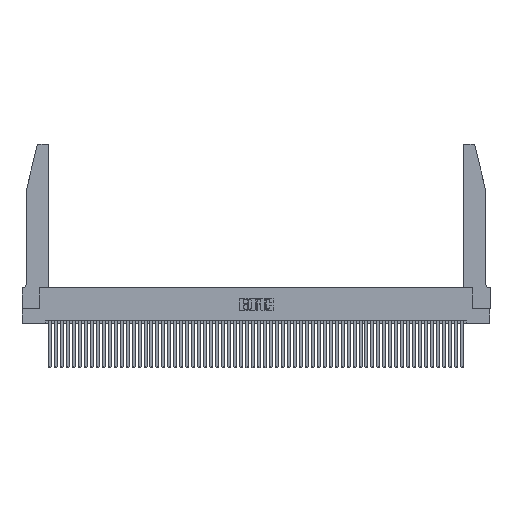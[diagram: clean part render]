
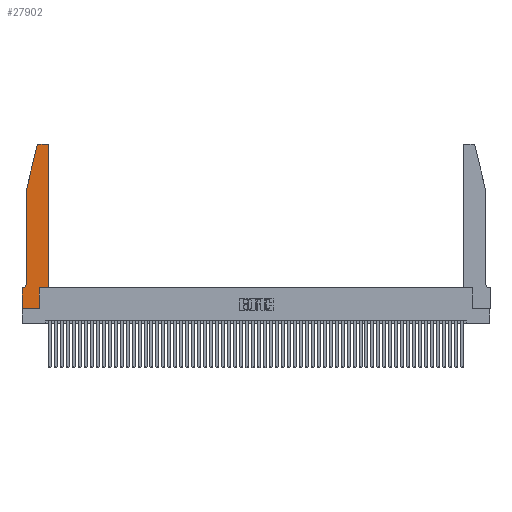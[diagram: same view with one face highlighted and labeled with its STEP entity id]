
A CAD part, top view. The second image highlights one B-rep face of the part: STEP entity #27902.
In plain terms, the highlighted planar face has unit normal (0, 0, 1).
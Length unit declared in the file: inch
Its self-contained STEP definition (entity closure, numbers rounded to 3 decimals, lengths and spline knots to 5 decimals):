
#57 = ORIENTED_EDGE ( 'NONE', *, *, #36650, .T. ) ;
#252 = DIRECTION ( 'NONE',  ( -1., 0., 0. ) ) ;
#535 = LINE ( 'NONE', #14785, #45060 ) ;
#554 = CARTESIAN_POINT ( 'NONE',  ( 0.284, 2.75, 0.37 ) ) ;
#903 = DIRECTION ( 'NONE',  ( 0., 0., 1. ) ) ;
#1165 = EDGE_CURVE ( 'NONE', #12063, #47447, #8140, .T. ) ;
#1200 = CARTESIAN_POINT ( 'NONE',  ( 0.0755, 2., 0.37 ) ) ;
#1361 = CARTESIAN_POINT ( 'NONE',  ( 0., 0.35, 0.37 ) ) ;
#1386 = FACE_OUTER_BOUND ( 'NONE', #52553, .T. ) ;
#3301 = DIRECTION ( 'NONE',  ( -1., 0., 0. ) ) ;
#3852 = CARTESIAN_POINT ( 'NONE',  ( 0.4505, 0.35, 0.37 ) ) ;
#4011 = VERTEX_POINT ( 'NONE', #37420 ) ;
#4111 = EDGE_CURVE ( 'NONE', #13767, #12063, #19401, .T. ) ;
#4223 = CARTESIAN_POINT ( 'NONE',  ( 0.0055, 0.35, 0.37 ) ) ;
#5656 = CARTESIAN_POINT ( 'NONE',  ( 0.2865, 0.35, 0.37 ) ) ;
#5822 = LINE ( 'NONE', #30712, #37590 ) ;
#6964 = VECTOR ( 'NONE', #34109, 39.37008 ) ;
#7444 = EDGE_CURVE ( 'NONE', #44826, #19031, #23081, .T. ) ;
#7683 = DIRECTION ( 'NONE',  ( 0., 0., 1. ) ) ;
#7916 = DIRECTION ( 'NONE',  ( 0., -1., 0. ) ) ;
#8140 = CIRCLE ( 'NONE', #15231, 0.03 ) ;
#8485 = DIRECTION ( 'NONE',  ( 0., 0., 1. ) ) ;
#9346 = ORIENTED_EDGE ( 'NONE', *, *, #47945, .T. ) ;
#9881 = LINE ( 'NONE', #29501, #21420 ) ;
#10178 = VECTOR ( 'NONE', #25687, 39.37008 ) ;
#10452 = VERTEX_POINT ( 'NONE', #23233 ) ;
#10533 = CIRCLE ( 'NONE', #49931, 0.03 ) ;
#10679 = CARTESIAN_POINT ( 'NONE',  ( 0.0755, 0.42, 0.37 ) ) ;
#11025 = LINE ( 'NONE', #46270, #55448 ) ;
#11802 = CARTESIAN_POINT ( 'NONE',  ( 0.4205, 2.75, 0.37 ) ) ;
#11993 = VERTEX_POINT ( 'NONE', #34749 ) ;
#12063 = VERTEX_POINT ( 'NONE', #554 ) ;
#13767 = VERTEX_POINT ( 'NONE', #11802 ) ;
#14785 = CARTESIAN_POINT ( 'NONE',  ( 0.4505, 0.35, 0.37 ) ) ;
#14830 = ORIENTED_EDGE ( 'NONE', *, *, #38845, .T. ) ;
#15144 = AXIS2_PLACEMENT_3D ( 'NONE', #34397, #8485, #38684 ) ;
#15231 = AXIS2_PLACEMENT_3D ( 'NONE', #33603, #7683, #37919 ) ;
#15746 = CARTESIAN_POINT ( 'NONE',  ( 0.4505, 2.72, 0.37 ) ) ;
#16103 = ORIENTED_EDGE ( 'NONE', *, *, #24331, .T. ) ;
#16432 = ORIENTED_EDGE ( 'NONE', *, *, #1165, .T. ) ;
#16572 = VECTOR ( 'NONE', #23095, 39.37008 ) ;
#19006 = ORIENTED_EDGE ( 'NONE', *, *, #34104, .T. ) ;
#19031 = VERTEX_POINT ( 'NONE', #29250 ) ;
#19401 = LINE ( 'NONE', #50860, #50999 ) ;
#20059 = EDGE_CURVE ( 'NONE', #19031, #11993, #28097, .T. ) ;
#21118 = EDGE_CURVE ( 'NONE', #48127, #44826, #11025, .T. ) ;
#21420 = VECTOR ( 'NONE', #7916, 39.37008 ) ;
#23081 = LINE ( 'NONE', #25513, #10178 ) ;
#23095 = DIRECTION ( 'NONE',  ( 0., 1., 0. ) ) ;
#23233 = CARTESIAN_POINT ( 'NONE',  ( 0.4505, 0.35, 0.37 ) ) ;
#23531 = DIRECTION ( 'NONE',  ( 1., 0., 0. ) ) ;
#23615 = VECTOR ( 'NONE', #48489, 39.37008 ) ;
#24331 = EDGE_CURVE ( 'NONE', #11993, #10452, #535, .T. ) ;
#25513 = CARTESIAN_POINT ( 'NONE',  ( 0., 0., 0.37 ) ) ;
#25687 = DIRECTION ( 'NONE',  ( 1., 0., 0. ) ) ;
#25731 = PLANE ( 'NONE',  #15144 ) ;
#26732 = VERTEX_POINT ( 'NONE', #10679 ) ;
#26828 = CARTESIAN_POINT ( 'NONE',  ( 0.4205, 2.72, 0.37 ) ) ;
#27902 = ADVANCED_FACE ( 'NONE', ( #1386 ), #25731, .T. ) ;
#28097 = LINE ( 'NONE', #5656, #16572 ) ;
#28155 = ORIENTED_EDGE ( 'NONE', *, *, #4111, .T. ) ;
#29241 = DIRECTION ( 'NONE',  ( 0., 0., -1. ) ) ;
#29250 = CARTESIAN_POINT ( 'NONE',  ( 0.2865, 0., 0.37 ) ) ;
#29501 = CARTESIAN_POINT ( 'NONE',  ( 0.0755, 2., 0.37 ) ) ;
#30712 = CARTESIAN_POINT ( 'NONE',  ( 0.0755, 0.35, 0.37 ) ) ;
#30975 = ORIENTED_EDGE ( 'NONE', *, *, #34367, .T. ) ;
#31174 = DIRECTION ( 'NONE',  ( 1., 0., 0. ) ) ;
#33179 = ORIENTED_EDGE ( 'NONE', *, *, #38537, .T. ) ;
#33603 = CARTESIAN_POINT ( 'NONE',  ( 0.284, 2.72, 0.37 ) ) ;
#34104 = EDGE_CURVE ( 'NONE', #4011, #26732, #9881, .T. ) ;
#34109 = DIRECTION ( 'NONE',  ( 0., 1., 0. ) ) ;
#34367 = EDGE_CURVE ( 'NONE', #51467, #13767, #10533, .T. ) ;
#34397 = CARTESIAN_POINT ( 'NONE',  ( 0., 0.35, 0.37 ) ) ;
#34749 = CARTESIAN_POINT ( 'NONE',  ( 0.2865, 0.35, 0.37 ) ) ;
#35050 = AXIS2_PLACEMENT_3D ( 'NONE', #54877, #29241, #3301 ) ;
#36427 = ORIENTED_EDGE ( 'NONE', *, *, #7444, .T. ) ;
#36650 = EDGE_CURVE ( 'NONE', #10452, #51467, #40038, .T. ) ;
#36732 = VERTEX_POINT ( 'NONE', #4223 ) ;
#37420 = CARTESIAN_POINT ( 'NONE',  ( 0.0755, 2., 0.37 ) ) ;
#37590 = VECTOR ( 'NONE', #252, 39.37008 ) ;
#37872 = DIRECTION ( 'NONE',  ( 0., -1., 0. ) ) ;
#37919 = DIRECTION ( 'NONE',  ( 1., 0., 0. ) ) ;
#38537 = EDGE_CURVE ( 'NONE', #26732, #36732, #41119, .T. ) ;
#38565 = CARTESIAN_POINT ( 'NONE',  ( 0., 0., 0.37 ) ) ;
#38684 = DIRECTION ( 'NONE',  ( 1., 0., 0. ) ) ;
#38845 = EDGE_CURVE ( 'NONE', #47447, #4011, #49117, .T. ) ;
#40038 = LINE ( 'NONE', #3852, #6964 ) ;
#40594 = ORIENTED_EDGE ( 'NONE', *, *, #20059, .T. ) ;
#40670 = CARTESIAN_POINT ( 'NONE',  ( 0.25487, 2.72718, 0.37 ) ) ;
#41119 = CIRCLE ( 'NONE', #35050, 0.07 ) ;
#42264 = DIRECTION ( 'NONE',  ( -1., 0., 0. ) ) ;
#44725 = ORIENTED_EDGE ( 'NONE', *, *, #21118, .T. ) ;
#44826 = VERTEX_POINT ( 'NONE', #38565 ) ;
#45060 = VECTOR ( 'NONE', #23531, 39.37008 ) ;
#46270 = CARTESIAN_POINT ( 'NONE',  ( 0., 0., 0.37 ) ) ;
#47447 = VERTEX_POINT ( 'NONE', #40670 ) ;
#47945 = EDGE_CURVE ( 'NONE', #36732, #48127, #5822, .T. ) ;
#48127 = VERTEX_POINT ( 'NONE', #1361 ) ;
#48489 = DIRECTION ( 'NONE',  ( -0.239, -0.971, 0. ) ) ;
#49117 = LINE ( 'NONE', #1200, #23615 ) ;
#49931 = AXIS2_PLACEMENT_3D ( 'NONE', #26828, #903, #31174 ) ;
#50860 = CARTESIAN_POINT ( 'NONE',  ( 0.2605, 2.75, 0.37 ) ) ;
#50999 = VECTOR ( 'NONE', #42264, 39.37008 ) ;
#51467 = VERTEX_POINT ( 'NONE', #15746 ) ;
#52553 = EDGE_LOOP ( 'NONE', ( #28155, #16432, #14830, #19006, #33179, #9346, #44725, #36427, #40594, #16103, #57, #30975 ) ) ;
#54877 = CARTESIAN_POINT ( 'NONE',  ( 0.0055, 0.42, 0.37 ) ) ;
#55448 = VECTOR ( 'NONE', #37872, 39.37008 ) ;
